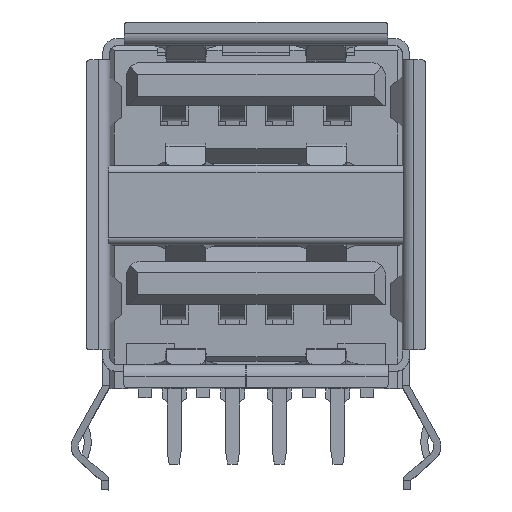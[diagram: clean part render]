
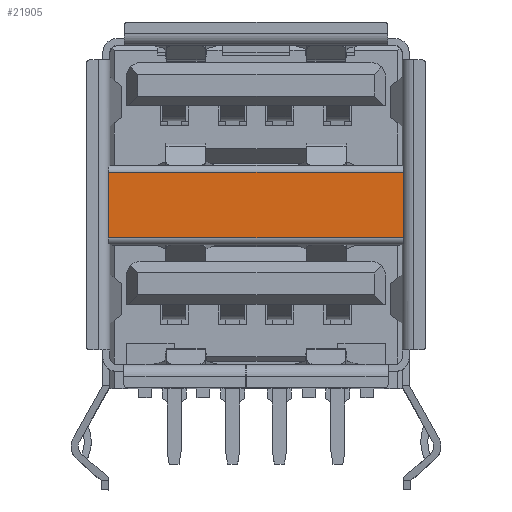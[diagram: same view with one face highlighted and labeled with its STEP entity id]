
A CAD part, top view. The second image highlights one B-rep face of the part: STEP entity #21905.
In plain terms, the highlighted planar face has unit normal (0, 0, 1).
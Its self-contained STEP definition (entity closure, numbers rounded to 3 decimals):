
#379 = DIRECTION ( 'NONE',  ( 0., 0., 1. ) ) ;
#3186 = EDGE_CURVE ( 'NONE', #25263, #44148, #39124, .T. ) ;
#3996 = CARTESIAN_POINT ( 'NONE',  ( -11.834, 7.778, 28.26 ) ) ;
#5871 = VECTOR ( 'NONE', #37560, 1000. ) ;
#8253 = EDGE_CURVE ( 'NONE', #44148, #11369, #14892, .T. ) ;
#8837 = LINE ( 'NONE', #26556, #5871 ) ;
#8957 = VECTOR ( 'NONE', #10171, 1000. ) ;
#10171 = DIRECTION ( 'NONE',  ( 0., -1., 0. ) ) ;
#10892 = CARTESIAN_POINT ( 'NONE',  ( -11.834, 4.978, 28.26 ) ) ;
#11369 = VERTEX_POINT ( 'NONE', #12117 ) ;
#11760 = DIRECTION ( 'NONE',  ( 0., -1., 0. ) ) ;
#12117 = CARTESIAN_POINT ( 'NONE',  ( 0.766, 4.978, 28.26 ) ) ;
#12334 = AXIS2_PLACEMENT_3D ( 'NONE', #35575, #379, #43934 ) ;
#14892 = LINE ( 'NONE', #29463, #21391 ) ;
#16638 = ORIENTED_EDGE ( 'NONE', *, *, #27463, .F. ) ;
#16723 = EDGE_CURVE ( 'NONE', #25263, #19741, #8837, .T. ) ;
#19175 = ORIENTED_EDGE ( 'NONE', *, *, #8253, .T. ) ;
#19741 = VERTEX_POINT ( 'NONE', #33795 ) ;
#21003 = PLANE ( 'NONE',  #12334 ) ;
#21391 = VECTOR ( 'NONE', #32579, 1000. ) ;
#21905 = ADVANCED_FACE ( 'NONE', ( #31758 ), #21003, .T. ) ;
#25263 = VERTEX_POINT ( 'NONE', #3996 ) ;
#25892 = LINE ( 'NONE', #29708, #31771 ) ;
#26556 = CARTESIAN_POINT ( 'NONE',  ( -12.086, 7.778, 28.26 ) ) ;
#27463 = EDGE_CURVE ( 'NONE', #19741, #11369, #25892, .T. ) ;
#29463 = CARTESIAN_POINT ( 'NONE',  ( -5.534, 4.978, 28.26 ) ) ;
#29708 = CARTESIAN_POINT ( 'NONE',  ( 0.766, 6.378, 28.26 ) ) ;
#31758 = FACE_OUTER_BOUND ( 'NONE', #37844, .T. ) ;
#31771 = VECTOR ( 'NONE', #11760, 1000. ) ;
#31980 = ORIENTED_EDGE ( 'NONE', *, *, #3186, .T. ) ;
#32579 = DIRECTION ( 'NONE',  ( 1., 0., 0. ) ) ;
#33795 = CARTESIAN_POINT ( 'NONE',  ( 0.766, 7.778, 28.26 ) ) ;
#35491 = ORIENTED_EDGE ( 'NONE', *, *, #16723, .F. ) ;
#35575 = CARTESIAN_POINT ( 'NONE',  ( -5.534, 6.378, 28.26 ) ) ;
#37560 = DIRECTION ( 'NONE',  ( 1., 0., 0. ) ) ;
#37844 = EDGE_LOOP ( 'NONE', ( #31980, #19175, #16638, #35491 ) ) ;
#39124 = LINE ( 'NONE', #46780, #8957 ) ;
#43934 = DIRECTION ( 'NONE',  ( 1., 0., 0. ) ) ;
#44148 = VERTEX_POINT ( 'NONE', #10892 ) ;
#46780 = CARTESIAN_POINT ( 'NONE',  ( -11.834, 6.378, 28.26 ) ) ;
